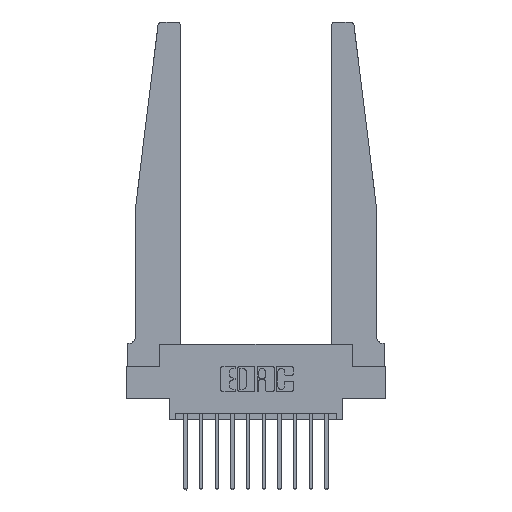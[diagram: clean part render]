
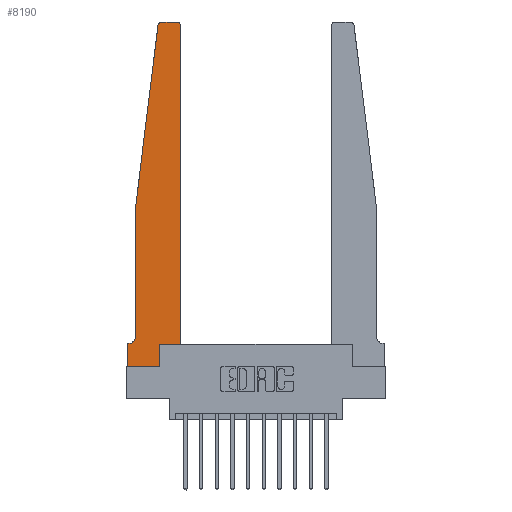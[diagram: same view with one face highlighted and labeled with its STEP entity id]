
A CAD part, top view. The second image highlights one B-rep face of the part: STEP entity #8190.
In plain terms, the highlighted planar face has unit normal (0, 0, 1).
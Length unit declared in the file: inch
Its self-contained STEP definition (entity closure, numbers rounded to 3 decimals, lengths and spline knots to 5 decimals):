
#37 = CARTESIAN_POINT ( 'NONE',  ( 0.015, 0.2375, 0.37 ) ) ;
#266 = CARTESIAN_POINT ( 'NONE',  ( 0.27653, 2.72, 0.37 ) ) ;
#457 = CARTESIAN_POINT ( 'NONE',  ( 0.065, 0.2375, 0.37 ) ) ;
#549 = LINE ( 'NONE', #8247, #3771 ) ;
#840 = ORIENTED_EDGE ( 'NONE', *, *, #14249, .T. ) ;
#956 = VERTEX_POINT ( 'NONE', #2796 ) ;
#1038 = EDGE_CURVE ( 'NONE', #956, #14401, #2808, .T. ) ;
#1070 = CARTESIAN_POINT ( 'NONE',  ( 0.395, 2.72, 0.37 ) ) ;
#1158 = CARTESIAN_POINT ( 'NONE',  ( 0., 0., 0.37 ) ) ;
#1292 = EDGE_CURVE ( 'NONE', #14401, #3297, #12267, .T. ) ;
#1359 = DIRECTION ( 'NONE',  ( -1., 0., 0. ) ) ;
#1364 = CARTESIAN_POINT ( 'NONE',  ( 0.015, 0.1875, 0.37 ) ) ;
#1452 = LINE ( 'NONE', #4920, #13939 ) ;
#1563 = DIRECTION ( 'NONE',  ( 1., 0., 0. ) ) ;
#1943 = ORIENTED_EDGE ( 'NONE', *, *, #1038, .T. ) ;
#2118 = CARTESIAN_POINT ( 'NONE',  ( 0.065, 1.25, 0.37 ) ) ;
#2288 = DIRECTION ( 'NONE',  ( 1., 0., 0. ) ) ;
#2464 = EDGE_CURVE ( 'NONE', #13108, #14840, #1452, .T. ) ;
#2569 = ORIENTED_EDGE ( 'NONE', *, *, #5618, .T. ) ;
#2587 = AXIS2_PLACEMENT_3D ( 'NONE', #1070, #9547, #2288 ) ;
#2796 = CARTESIAN_POINT ( 'NONE',  ( 0.24675, 2.72367, 0.37 ) ) ;
#2808 = LINE ( 'NONE', #5349, #15301 ) ;
#2881 = VECTOR ( 'NONE', #3588, 39.37008 ) ;
#3297 = VERTEX_POINT ( 'NONE', #457 ) ;
#3324 = LINE ( 'NONE', #4384, #9383 ) ;
#3415 = DIRECTION ( 'NONE',  ( 0., -1., 0. ) ) ;
#3454 = VECTOR ( 'NONE', #13749, 39.37008 ) ;
#3588 = DIRECTION ( 'NONE',  ( 1., 0., 0. ) ) ;
#3771 = VECTOR ( 'NONE', #15481, 39.37008 ) ;
#4179 = CARTESIAN_POINT ( 'NONE',  ( 0.2605, 0.18, 0.37 ) ) ;
#4384 = CARTESIAN_POINT ( 'NONE',  ( 0., 0., 0.37 ) ) ;
#4418 = CARTESIAN_POINT ( 'NONE',  ( 0.425, 0.18, 0.37 ) ) ;
#4920 = CARTESIAN_POINT ( 'NONE',  ( 0.425, 0.18, 0.37 ) ) ;
#5201 = EDGE_CURVE ( 'NONE', #13049, #956, #8572, .T. ) ;
#5349 = CARTESIAN_POINT ( 'NONE',  ( 0.065, 1.25, 0.37 ) ) ;
#5505 = PLANE ( 'NONE',  #9489 ) ;
#5605 = CARTESIAN_POINT ( 'NONE',  ( 0., 0., 0.37 ) ) ;
#5618 = EDGE_CURVE ( 'NONE', #6584, #6434, #9703, .T. ) ;
#5798 = ORIENTED_EDGE ( 'NONE', *, *, #5201, .T. ) ;
#5958 = CARTESIAN_POINT ( 'NONE',  ( 0., 0.1875, 0.37 ) ) ;
#6204 = VECTOR ( 'NONE', #3415, 39.37008 ) ;
#6346 = CIRCLE ( 'NONE', #2587, 0.03 ) ;
#6434 = VERTEX_POINT ( 'NONE', #10238 ) ;
#6507 = CARTESIAN_POINT ( 'NONE',  ( 0.2605, 0.18, 0.37 ) ) ;
#6584 = VERTEX_POINT ( 'NONE', #5605 ) ;
#6701 = EDGE_CURVE ( 'NONE', #9986, #15064, #549, .T. ) ;
#6728 = DIRECTION ( 'NONE',  ( 0., 0., 1. ) ) ;
#6805 = EDGE_CURVE ( 'NONE', #10744, #13049, #8709, .T. ) ;
#7102 = ORIENTED_EDGE ( 'NONE', *, *, #10411, .T. ) ;
#7276 = ORIENTED_EDGE ( 'NONE', *, *, #14023, .T. ) ;
#7813 = EDGE_LOOP ( 'NONE', ( #9804, #5798, #1943, #9756, #7276, #10066, #12812, #2569, #13930, #11352, #840, #7102 ) ) ;
#8159 = AXIS2_PLACEMENT_3D ( 'NONE', #266, #8800, #1563 ) ;
#8190 = ADVANCED_FACE ( 'NONE', ( #13038 ), #5505, .T. ) ;
#8247 = CARTESIAN_POINT ( 'NONE',  ( 0.065, 0.1875, 0.37 ) ) ;
#8572 = CIRCLE ( 'NONE', #8159, 0.03 ) ;
#8595 = DIRECTION ( 'NONE',  ( 0., 0., -1. ) ) ;
#8609 = CIRCLE ( 'NONE', #13071, 0.05 ) ;
#8709 = LINE ( 'NONE', #11999, #11943 ) ;
#8800 = DIRECTION ( 'NONE',  ( 0., 0., 1. ) ) ;
#9383 = VECTOR ( 'NONE', #12868, 39.37008 ) ;
#9489 = AXIS2_PLACEMENT_3D ( 'NONE', #13966, #6728, #15179 ) ;
#9547 = DIRECTION ( 'NONE',  ( 0., 0., 1. ) ) ;
#9658 = EDGE_CURVE ( 'NONE', #15064, #6584, #3324, .T. ) ;
#9703 = LINE ( 'NONE', #1158, #2881 ) ;
#9756 = ORIENTED_EDGE ( 'NONE', *, *, #1292, .T. ) ;
#9772 = DIRECTION ( 'NONE',  ( -1., 0., 0. ) ) ;
#9804 = ORIENTED_EDGE ( 'NONE', *, *, #6805, .T. ) ;
#9986 = VERTEX_POINT ( 'NONE', #1364 ) ;
#10066 = ORIENTED_EDGE ( 'NONE', *, *, #6701, .T. ) ;
#10238 = CARTESIAN_POINT ( 'NONE',  ( 0.2605, 0., 0.37 ) ) ;
#10256 = CARTESIAN_POINT ( 'NONE',  ( 0.395, 2.75, 0.37 ) ) ;
#10411 = EDGE_CURVE ( 'NONE', #11951, #10744, #6346, .T. ) ;
#10683 = CARTESIAN_POINT ( 'NONE',  ( 0.065, 1.25, 0.37 ) ) ;
#10744 = VERTEX_POINT ( 'NONE', #10256 ) ;
#11287 = VECTOR ( 'NONE', #11685, 39.37008 ) ;
#11348 = CARTESIAN_POINT ( 'NONE',  ( 0.27653, 2.75, 0.37 ) ) ;
#11352 = ORIENTED_EDGE ( 'NONE', *, *, #2464, .T. ) ;
#11409 = EDGE_CURVE ( 'NONE', #6434, #13108, #12771, .T. ) ;
#11595 = CARTESIAN_POINT ( 'NONE',  ( 0.425, 2.72, 0.37 ) ) ;
#11685 = DIRECTION ( 'NONE',  ( 0., 1., 0. ) ) ;
#11943 = VECTOR ( 'NONE', #9772, 39.37008 ) ;
#11951 = VERTEX_POINT ( 'NONE', #11595 ) ;
#11999 = CARTESIAN_POINT ( 'NONE',  ( 0.25, 2.75, 0.37 ) ) ;
#12267 = LINE ( 'NONE', #10683, #6204 ) ;
#12596 = DIRECTION ( 'NONE',  ( -0.122, -0.992, 0. ) ) ;
#12771 = LINE ( 'NONE', #6507, #3454 ) ;
#12812 = ORIENTED_EDGE ( 'NONE', *, *, #9658, .T. ) ;
#12868 = DIRECTION ( 'NONE',  ( 0., -1., 0. ) ) ;
#13038 = FACE_OUTER_BOUND ( 'NONE', #7813, .T. ) ;
#13049 = VERTEX_POINT ( 'NONE', #11348 ) ;
#13071 = AXIS2_PLACEMENT_3D ( 'NONE', #37, #8595, #1359 ) ;
#13108 = VERTEX_POINT ( 'NONE', #4179 ) ;
#13746 = CARTESIAN_POINT ( 'NONE',  ( 0.425, 0.18, 0.37 ) ) ;
#13749 = DIRECTION ( 'NONE',  ( 0., 1., 0. ) ) ;
#13930 = ORIENTED_EDGE ( 'NONE', *, *, #11409, .T. ) ;
#13939 = VECTOR ( 'NONE', #14585, 39.37008 ) ;
#13966 = CARTESIAN_POINT ( 'NONE',  ( 0., 0.1875, 0.37 ) ) ;
#14023 = EDGE_CURVE ( 'NONE', #3297, #9986, #8609, .T. ) ;
#14249 = EDGE_CURVE ( 'NONE', #14840, #11951, #14863, .T. ) ;
#14401 = VERTEX_POINT ( 'NONE', #2118 ) ;
#14585 = DIRECTION ( 'NONE',  ( 1., 0., 0. ) ) ;
#14840 = VERTEX_POINT ( 'NONE', #13746 ) ;
#14863 = LINE ( 'NONE', #4418, #11287 ) ;
#15064 = VERTEX_POINT ( 'NONE', #5958 ) ;
#15179 = DIRECTION ( 'NONE',  ( 1., 0., 0. ) ) ;
#15301 = VECTOR ( 'NONE', #12596, 39.37008 ) ;
#15481 = DIRECTION ( 'NONE',  ( -1., 0., 0. ) ) ;
